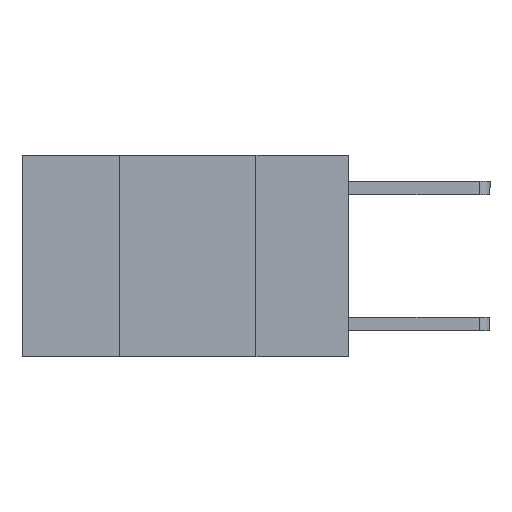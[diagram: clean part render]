
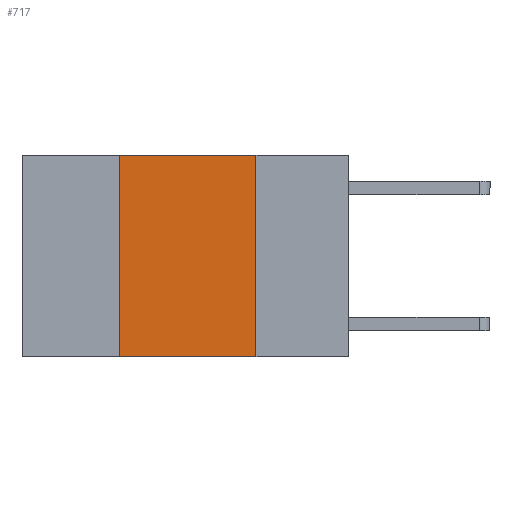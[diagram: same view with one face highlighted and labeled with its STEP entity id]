
A CAD part, left-side view. The second image highlights one B-rep face of the part: STEP entity #717.
In plain terms, the highlighted planar face has unit normal (-1, 0, 0).
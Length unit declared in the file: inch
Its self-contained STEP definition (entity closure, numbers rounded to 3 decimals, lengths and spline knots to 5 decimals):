
#35 = PLANE ( 'NONE',  #3931 ) ;
#474 = VECTOR ( 'NONE', #5282, 39.37008 ) ;
#521 = LINE ( 'NONE', #3874, #4501 ) ;
#617 = FACE_OUTER_BOUND ( 'NONE', #3546, .T. ) ;
#665 = DIRECTION ( 'NONE',  ( 1., 0., 0. ) ) ;
#717 = ADVANCED_FACE ( 'NONE', ( #617 ), #35, .F. ) ;
#814 = CARTESIAN_POINT ( 'NONE',  ( 0., 0.42, 0. ) ) ;
#894 = EDGE_CURVE ( 'NONE', #1499, #4173, #521, .T. ) ;
#1115 = CARTESIAN_POINT ( 'NONE',  ( 0., 0.17, 0. ) ) ;
#1282 = ORIENTED_EDGE ( 'NONE', *, *, #5440, .F. ) ;
#1499 = VERTEX_POINT ( 'NONE', #7577 ) ;
#2451 = DIRECTION ( 'NONE',  ( 0., 0., -1. ) ) ;
#3078 = ORIENTED_EDGE ( 'NONE', *, *, #894, .T. ) ;
#3147 = DIRECTION ( 'NONE',  ( 0., -1., 0. ) ) ;
#3177 = VECTOR ( 'NONE', #3411, 39.37008 ) ;
#3222 = LINE ( 'NONE', #7826, #474 ) ;
#3331 = CARTESIAN_POINT ( 'NONE',  ( 0., 0.17, 0. ) ) ;
#3411 = DIRECTION ( 'NONE',  ( 0., 0., 1. ) ) ;
#3546 = EDGE_LOOP ( 'NONE', ( #4306, #1282, #6010, #3078 ) ) ;
#3874 = CARTESIAN_POINT ( 'NONE',  ( 0., 0.6, -0.37 ) ) ;
#3931 = AXIS2_PLACEMENT_3D ( 'NONE', #4689, #665, #6198 ) ;
#4173 = VERTEX_POINT ( 'NONE', #6157 ) ;
#4306 = ORIENTED_EDGE ( 'NONE', *, *, #5109, .F. ) ;
#4346 = CARTESIAN_POINT ( 'NONE',  ( 0., 0.42, 0. ) ) ;
#4501 = VECTOR ( 'NONE', #3147, 39.37008 ) ;
#4532 = VECTOR ( 'NONE', #2451, 39.37008 ) ;
#4689 = CARTESIAN_POINT ( 'NONE',  ( 0., 0.6, 0. ) ) ;
#5109 = EDGE_CURVE ( 'NONE', #8607, #4173, #7280, .T. ) ;
#5282 = DIRECTION ( 'NONE',  ( 0., -1., 0. ) ) ;
#5440 = EDGE_CURVE ( 'NONE', #6402, #8607, #3222, .T. ) ;
#6010 = ORIENTED_EDGE ( 'NONE', *, *, #6635, .F. ) ;
#6157 = CARTESIAN_POINT ( 'NONE',  ( 0., 0.17, -0.37 ) ) ;
#6198 = DIRECTION ( 'NONE',  ( 0., 0., -1. ) ) ;
#6402 = VERTEX_POINT ( 'NONE', #4346 ) ;
#6635 = EDGE_CURVE ( 'NONE', #1499, #6402, #7471, .T. ) ;
#7280 = LINE ( 'NONE', #1115, #4532 ) ;
#7471 = LINE ( 'NONE', #814, #3177 ) ;
#7577 = CARTESIAN_POINT ( 'NONE',  ( 0., 0.42, -0.37 ) ) ;
#7826 = CARTESIAN_POINT ( 'NONE',  ( 0., 0.6, 0. ) ) ;
#8607 = VERTEX_POINT ( 'NONE', #3331 ) ;
